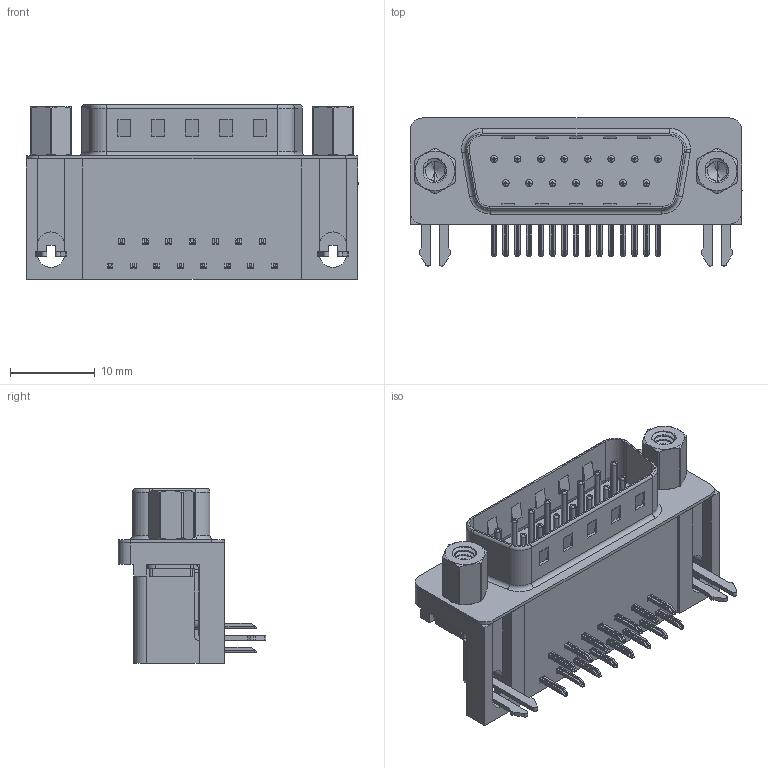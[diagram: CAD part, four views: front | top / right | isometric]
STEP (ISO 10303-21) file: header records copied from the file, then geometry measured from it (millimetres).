
FILE_DESCRIPTION (( 'STEP AP203' ), '1' );
FILE_NAME ('629-015-340-033.STEP', '2021-09-21T20:13:25', ( '' ), ( '' ), 'SwSTEP 2.0', 'SolidWorks 2020', '' );
FILE_SCHEMA (( 'CONFIG_CONTROL_DESIGN' ));
Length unit declared in the file: millimetre
Products named in the file (8): 629 4-40 Hex Standoff 5; 629 Contact Top; 629 Housing_15 Socket; 629 Contact Bottom; 629 4-40 Threaded Rivet; 629-015-340-033; 629 Shell_15 Socket; 629 2 Prong Board Lock
Assembly tree (23 placements, depth 2):
  629-015-340-033
    629 Housing_15 Socket
    629 Shell_15 Socket
    629 Contact Bottom  x7
    629 Contact Top  x8
    629 2 Prong Board Lock  x2
    629 4-40 Threaded Rivet  x2
    629 4-40 Hex Standoff 5  x2
Bounding box: 39.22 x 17.48 x 20.6 mm (x, y, z)
Volume: 5293.6 mm3; surface area: 6561.4 mm2
Topology: 23 solids, 23 shells, 1641 faces, 4141 edges, 2583 vertices
Faces by surface type: plane 945, cylinder 525, torus 121, cone 32, bspline 18
Entity records: 24324 total; most frequent: CARTESIAN_POINT 7927, ORIENTED_EDGE 3162, DIRECTION 3143, EDGE_CURVE 1581, AXIS2_PLACEMENT_3D 1061, VECTOR 1021, LINE 1021, VERTEX_POINT 1014
